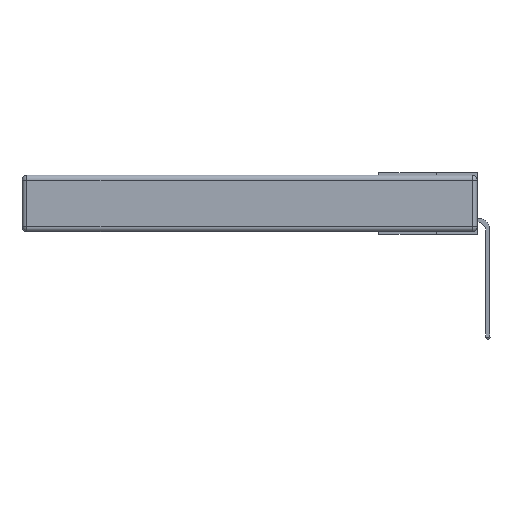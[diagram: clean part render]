
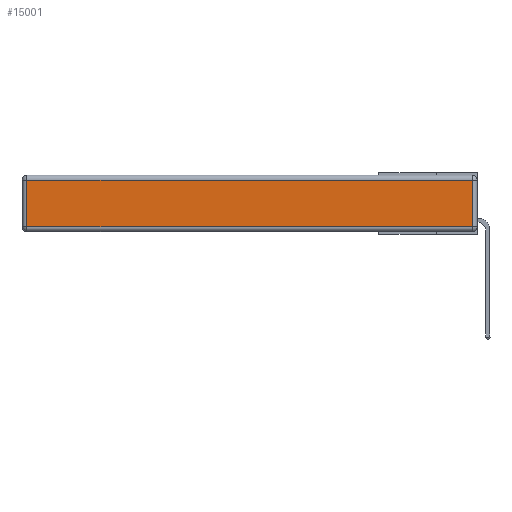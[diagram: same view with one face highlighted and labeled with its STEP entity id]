
A CAD part, left-side view. The second image highlights one B-rep face of the part: STEP entity #15001.
In plain terms, the highlighted planar face has unit normal (-1, 0, 0).
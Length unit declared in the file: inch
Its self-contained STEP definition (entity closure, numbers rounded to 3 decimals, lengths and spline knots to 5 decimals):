
#355 = DIRECTION ( 'NONE',  ( 0., 0., 1. ) ) ;
#363 = DIRECTION ( 'NONE',  ( 0., 0., 1. ) ) ;
#768 = VERTEX_POINT ( 'NONE', #2969 ) ;
#1071 = VERTEX_POINT ( 'NONE', #8708 ) ;
#1555 = VERTEX_POINT ( 'NONE', #4950 ) ;
#1672 = DIRECTION ( 'NONE',  ( 0., -1., 0. ) ) ;
#1774 = CARTESIAN_POINT ( 'NONE',  ( 0., 2.72, -0.343 ) ) ;
#2076 = VECTOR ( 'NONE', #2745, 39.37008 ) ;
#2745 = DIRECTION ( 'NONE',  ( 0., 1., 0. ) ) ;
#2969 = CARTESIAN_POINT ( 'NONE',  ( 0., 0.03, -0.03 ) ) ;
#3701 = ORIENTED_EDGE ( 'NONE', *, *, #8605, .T. ) ;
#4040 = LINE ( 'NONE', #14213, #2076 ) ;
#4194 = DIRECTION ( 'NONE',  ( 0., 0., -1. ) ) ;
#4950 = CARTESIAN_POINT ( 'NONE',  ( 0., 0.03, -0.313 ) ) ;
#5448 = LINE ( 'NONE', #14280, #8126 ) ;
#7784 = EDGE_LOOP ( 'NONE', ( #13147, #12240, #11609, #3701 ) ) ;
#7846 = LINE ( 'NONE', #9579, #11659 ) ;
#7888 = VECTOR ( 'NONE', #4194, 39.37008 ) ;
#8126 = VECTOR ( 'NONE', #1672, 39.37008 ) ;
#8276 = CARTESIAN_POINT ( 'NONE',  ( 0., 2.72, -0.313 ) ) ;
#8486 = PLANE ( 'NONE',  #11434 ) ;
#8605 = EDGE_CURVE ( 'NONE', #1071, #11416, #14063, .T. ) ;
#8677 = FACE_OUTER_BOUND ( 'NONE', #7784, .T. ) ;
#8708 = CARTESIAN_POINT ( 'NONE',  ( 0., 2.72, -0.03 ) ) ;
#9579 = CARTESIAN_POINT ( 'NONE',  ( 0., 0.03, -0.343 ) ) ;
#11416 = VERTEX_POINT ( 'NONE', #8276 ) ;
#11434 = AXIS2_PLACEMENT_3D ( 'NONE', #12001, #13155, #355 ) ;
#11609 = ORIENTED_EDGE ( 'NONE', *, *, #12649, .T. ) ;
#11659 = VECTOR ( 'NONE', #363, 39.37008 ) ;
#12001 = CARTESIAN_POINT ( 'NONE',  ( 0., 0., -0.343 ) ) ;
#12159 = EDGE_CURVE ( 'NONE', #1555, #768, #7846, .T. ) ;
#12240 = ORIENTED_EDGE ( 'NONE', *, *, #12159, .T. ) ;
#12649 = EDGE_CURVE ( 'NONE', #768, #1071, #4040, .T. ) ;
#13147 = ORIENTED_EDGE ( 'NONE', *, *, #14499, .T. ) ;
#13155 = DIRECTION ( 'NONE',  ( -1., 0., 0. ) ) ;
#14063 = LINE ( 'NONE', #1774, #7888 ) ;
#14213 = CARTESIAN_POINT ( 'NONE',  ( 0., 2.75, -0.03 ) ) ;
#14280 = CARTESIAN_POINT ( 'NONE',  ( 0., 0., -0.313 ) ) ;
#14499 = EDGE_CURVE ( 'NONE', #11416, #1555, #5448, .T. ) ;
#15001 = ADVANCED_FACE ( 'NONE', ( #8677 ), #8486, .T. ) ;
